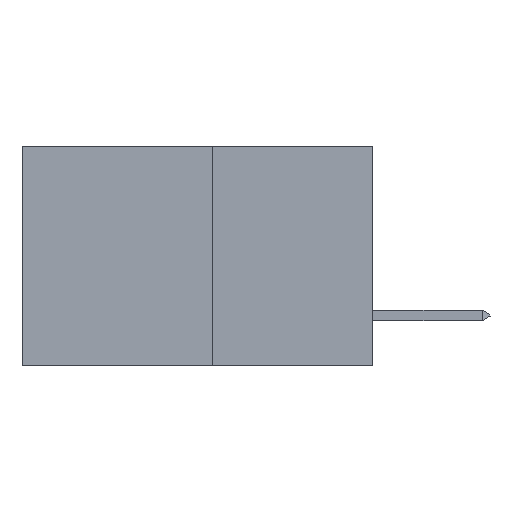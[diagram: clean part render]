
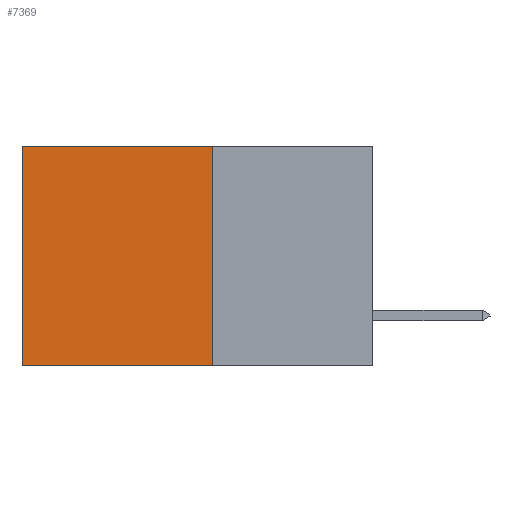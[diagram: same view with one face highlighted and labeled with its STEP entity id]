
A CAD part, left-side view. The second image highlights one B-rep face of the part: STEP entity #7369.
In plain terms, the highlighted planar face has unit normal (-1, 0, 0).
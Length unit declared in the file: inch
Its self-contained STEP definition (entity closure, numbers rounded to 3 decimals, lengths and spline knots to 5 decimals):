
#3455 = CARTESIAN_POINT ( 'NONE',  ( 0.277, 0.27, -0.37 ) ) ;
#4064 = CARTESIAN_POINT ( 'NONE',  ( 0.277, 0.59, -0.37 ) ) ;
#4316 = ORIENTED_EDGE ( 'NONE', *, *, #14186, .F. ) ;
#5534 = EDGE_CURVE ( 'NONE', #20214, #6079, #12885, .T. ) ;
#6079 = VERTEX_POINT ( 'NONE', #16031 ) ;
#7032 = DIRECTION ( 'NONE',  ( 0., 0., -1. ) ) ;
#7333 = ORIENTED_EDGE ( 'NONE', *, *, #14517, .F. ) ;
#7343 = VECTOR ( 'NONE', #21554, 39.37008 ) ;
#7369 = ADVANCED_FACE ( 'NONE', ( #14480 ), #19377, .F. ) ;
#7726 = VECTOR ( 'NONE', #14541, 39.37008 ) ;
#7760 = VERTEX_POINT ( 'NONE', #22095 ) ;
#8935 = DIRECTION ( 'NONE',  ( 1., 0., 0. ) ) ;
#9110 = VECTOR ( 'NONE', #13165, 39.37008 ) ;
#11910 = EDGE_CURVE ( 'NONE', #7760, #20214, #16611, .T. ) ;
#12120 = VECTOR ( 'NONE', #7032, 39.37008 ) ;
#12240 = ORIENTED_EDGE ( 'NONE', *, *, #11910, .T. ) ;
#12885 = LINE ( 'NONE', #4064, #7726 ) ;
#13165 = DIRECTION ( 'NONE',  ( 0., 1., 0. ) ) ;
#14186 = EDGE_CURVE ( 'NONE', #7760, #19611, #21424, .T. ) ;
#14480 = FACE_OUTER_BOUND ( 'NONE', #20373, .T. ) ;
#14517 = EDGE_CURVE ( 'NONE', #19611, #6079, #18363, .T. ) ;
#14541 = DIRECTION ( 'NONE',  ( 0., 0., -1. ) ) ;
#15856 = CARTESIAN_POINT ( 'NONE',  ( 0.277, 0.27, -0.37 ) ) ;
#16031 = CARTESIAN_POINT ( 'NONE',  ( 0.277, 0.59, -0.37 ) ) ;
#16611 = LINE ( 'NONE', #19811, #7343 ) ;
#16912 = CARTESIAN_POINT ( 'NONE',  ( 0.277, 0.27, -0.37 ) ) ;
#17121 = CARTESIAN_POINT ( 'NONE',  ( 0.277, 0.59, 0. ) ) ;
#18342 = CARTESIAN_POINT ( 'NONE',  ( 0.277, 0.27, -0.37 ) ) ;
#18363 = LINE ( 'NONE', #18342, #9110 ) ;
#19377 = PLANE ( 'NONE',  #22569 ) ;
#19611 = VERTEX_POINT ( 'NONE', #16912 ) ;
#19811 = CARTESIAN_POINT ( 'NONE',  ( 0.277, 0.27, 0. ) ) ;
#20214 = VERTEX_POINT ( 'NONE', #17121 ) ;
#20373 = EDGE_LOOP ( 'NONE', ( #21491, #7333, #4316, #12240 ) ) ;
#21139 = DIRECTION ( 'NONE',  ( 0., 0., -1. ) ) ;
#21424 = LINE ( 'NONE', #3455, #12120 ) ;
#21491 = ORIENTED_EDGE ( 'NONE', *, *, #5534, .T. ) ;
#21554 = DIRECTION ( 'NONE',  ( 0., 1., 0. ) ) ;
#22095 = CARTESIAN_POINT ( 'NONE',  ( 0.277, 0.27, 0. ) ) ;
#22569 = AXIS2_PLACEMENT_3D ( 'NONE', #15856, #8935, #21139 ) ;
